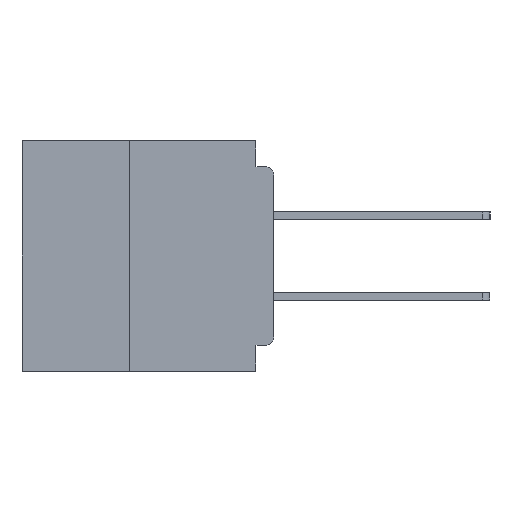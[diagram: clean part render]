
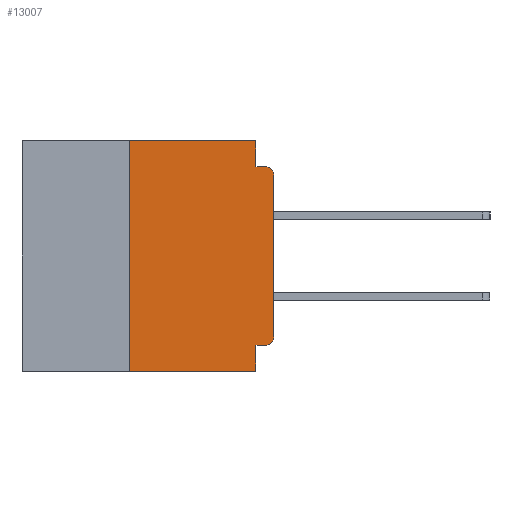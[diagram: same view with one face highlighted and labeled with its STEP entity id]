
A CAD part, left-side view. The second image highlights one B-rep face of the part: STEP entity #13007.
In plain terms, the highlighted planar face has unit normal (-1, 0, 0).
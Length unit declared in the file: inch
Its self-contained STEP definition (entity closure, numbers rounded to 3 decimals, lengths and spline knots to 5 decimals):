
#1230 = VECTOR ( 'NONE', #1669, 39.37008 ) ;
#1526 = VECTOR ( 'NONE', #24166, 39.37008 ) ;
#1539 = EDGE_CURVE ( 'NONE', #2088, #28704, #27056, .T. ) ;
#1577 = DIRECTION ( 'NONE',  ( 1., 0., 0. ) ) ;
#1669 = DIRECTION ( 'NONE',  ( 0., 0., -1. ) ) ;
#2088 = VERTEX_POINT ( 'NONE', #23785 ) ;
#2146 = LINE ( 'NONE', #23765, #1230 ) ;
#2412 = CARTESIAN_POINT ( 'NONE',  ( 0., 0.25, 0. ) ) ;
#3086 = CARTESIAN_POINT ( 'NONE',  ( 0., 0.437, 0. ) ) ;
#3230 = CARTESIAN_POINT ( 'NONE',  ( 0., 0.015, -0.06 ) ) ;
#4013 = ORIENTED_EDGE ( 'NONE', *, *, #7871, .T. ) ;
#4356 = EDGE_CURVE ( 'NONE', #7856, #13545, #13432, .T. ) ;
#4898 = CARTESIAN_POINT ( 'NONE',  ( 0., 0., -0.34 ) ) ;
#4908 = AXIS2_PLACEMENT_3D ( 'NONE', #5186, #5181, #5154 ) ;
#5154 = DIRECTION ( 'NONE',  ( 0., 0., -1. ) ) ;
#5181 = DIRECTION ( 'NONE',  ( -1., 0., 0. ) ) ;
#5186 = CARTESIAN_POINT ( 'NONE',  ( 0., 0.015, -0.34 ) ) ;
#5878 = VECTOR ( 'NONE', #6849, 39.37008 ) ;
#6099 = DIRECTION ( 'NONE',  ( 0., 0., -1. ) ) ;
#6849 = DIRECTION ( 'NONE',  ( 0., 0., -1. ) ) ;
#6973 = CARTESIAN_POINT ( 'NONE',  ( 0., 0.031, 0. ) ) ;
#7856 = VERTEX_POINT ( 'NONE', #31586 ) ;
#7871 = EDGE_CURVE ( 'NONE', #21757, #20809, #34379, .T. ) ;
#8032 = LINE ( 'NONE', #34534, #15504 ) ;
#8610 = ORIENTED_EDGE ( 'NONE', *, *, #1539, .F. ) ;
#8631 = VERTEX_POINT ( 'NONE', #18363 ) ;
#9402 = EDGE_CURVE ( 'NONE', #20416, #21757, #29729, .T. ) ;
#11066 = ORIENTED_EDGE ( 'NONE', *, *, #29482, .T. ) ;
#12129 = AXIS2_PLACEMENT_3D ( 'NONE', #15678, #1577, #21216 ) ;
#12743 = VECTOR ( 'NONE', #31195, 39.37008 ) ;
#13007 = ADVANCED_FACE ( 'NONE', ( #25629 ), #18445, .F. ) ;
#13432 = LINE ( 'NONE', #6973, #5878 ) ;
#13489 = ORIENTED_EDGE ( 'NONE', *, *, #29105, .F. ) ;
#13545 = VERTEX_POINT ( 'NONE', #33157 ) ;
#13551 = LINE ( 'NONE', #15366, #35156 ) ;
#14238 = EDGE_LOOP ( 'NONE', ( #4013, #11066, #13489, #27304, #28777, #8610, #14402, #28961, #27152, #27077 ) ) ;
#14402 = ORIENTED_EDGE ( 'NONE', *, *, #18350, .T. ) ;
#14555 = VECTOR ( 'NONE', #25350, 39.37008 ) ;
#15366 = CARTESIAN_POINT ( 'NONE',  ( 0., 0., -0.355 ) ) ;
#15504 = VECTOR ( 'NONE', #26480, 39.37008 ) ;
#15678 = CARTESIAN_POINT ( 'NONE',  ( 0., 0.437, 0. ) ) ;
#16155 = CARTESIAN_POINT ( 'NONE',  ( 0., 0.437, -0.4 ) ) ;
#16337 = CIRCLE ( 'NONE', #29214, 0.015 ) ;
#16557 = LINE ( 'NONE', #16155, #1526 ) ;
#17532 = EDGE_CURVE ( 'NONE', #20416, #22557, #13551, .T. ) ;
#18350 = EDGE_CURVE ( 'NONE', #2088, #30442, #16557, .T. ) ;
#18363 = CARTESIAN_POINT ( 'NONE',  ( 0., 0.015, -0.045 ) ) ;
#18445 = PLANE ( 'NONE',  #12129 ) ;
#19826 = VECTOR ( 'NONE', #26222, 39.37008 ) ;
#20416 = VERTEX_POINT ( 'NONE', #32063 ) ;
#20809 = VERTEX_POINT ( 'NONE', #28513 ) ;
#21216 = DIRECTION ( 'NONE',  ( 0., 0., -1. ) ) ;
#21757 = VERTEX_POINT ( 'NONE', #4898 ) ;
#22557 = VERTEX_POINT ( 'NONE', #35489 ) ;
#22776 = DIRECTION ( 'NONE',  ( -1., 0., 0. ) ) ;
#23765 = CARTESIAN_POINT ( 'NONE',  ( 0., 0.031, -0.4 ) ) ;
#23785 = CARTESIAN_POINT ( 'NONE',  ( 0., 0.25, -0.4 ) ) ;
#24128 = CARTESIAN_POINT ( 'NONE',  ( 0., 0.031, -0.4 ) ) ;
#24166 = DIRECTION ( 'NONE',  ( 0., -1., 0. ) ) ;
#25350 = DIRECTION ( 'NONE',  ( 0., -1., 0. ) ) ;
#25629 = FACE_OUTER_BOUND ( 'NONE', #14238, .T. ) ;
#26222 = DIRECTION ( 'NONE',  ( 0., 0., 1. ) ) ;
#26248 = CARTESIAN_POINT ( 'NONE',  ( 0., 0.25, -0.4 ) ) ;
#26480 = DIRECTION ( 'NONE',  ( 0., -1., 0. ) ) ;
#27056 = LINE ( 'NONE', #26248, #19826 ) ;
#27077 = ORIENTED_EDGE ( 'NONE', *, *, #9402, .T. ) ;
#27152 = ORIENTED_EDGE ( 'NONE', *, *, #17532, .F. ) ;
#27304 = ORIENTED_EDGE ( 'NONE', *, *, #4356, .F. ) ;
#28513 = CARTESIAN_POINT ( 'NONE',  ( 0., 0., -0.06 ) ) ;
#28704 = VERTEX_POINT ( 'NONE', #2412 ) ;
#28777 = ORIENTED_EDGE ( 'NONE', *, *, #35264, .F. ) ;
#28961 = ORIENTED_EDGE ( 'NONE', *, *, #30417, .F. ) ;
#29105 = EDGE_CURVE ( 'NONE', #13545, #8631, #8032, .T. ) ;
#29214 = AXIS2_PLACEMENT_3D ( 'NONE', #3230, #22776, #6099 ) ;
#29482 = EDGE_CURVE ( 'NONE', #20809, #8631, #16337, .T. ) ;
#29729 = CIRCLE ( 'NONE', #4908, 0.015 ) ;
#29865 = LINE ( 'NONE', #3086, #14555 ) ;
#30417 = EDGE_CURVE ( 'NONE', #22557, #30442, #2146, .T. ) ;
#30442 = VERTEX_POINT ( 'NONE', #24128 ) ;
#31147 = CARTESIAN_POINT ( 'NONE',  ( 0., 0., 0. ) ) ;
#31195 = DIRECTION ( 'NONE',  ( 0., 0., 1. ) ) ;
#31586 = CARTESIAN_POINT ( 'NONE',  ( 0., 0.031, 0. ) ) ;
#32063 = CARTESIAN_POINT ( 'NONE',  ( 0., 0.015, -0.355 ) ) ;
#33157 = CARTESIAN_POINT ( 'NONE',  ( 0., 0.031, -0.045 ) ) ;
#34302 = DIRECTION ( 'NONE',  ( 0., 1., 0. ) ) ;
#34379 = LINE ( 'NONE', #31147, #12743 ) ;
#34534 = CARTESIAN_POINT ( 'NONE',  ( 0., 0., -0.045 ) ) ;
#35156 = VECTOR ( 'NONE', #34302, 39.37008 ) ;
#35264 = EDGE_CURVE ( 'NONE', #28704, #7856, #29865, .T. ) ;
#35489 = CARTESIAN_POINT ( 'NONE',  ( 0., 0.031, -0.355 ) ) ;
